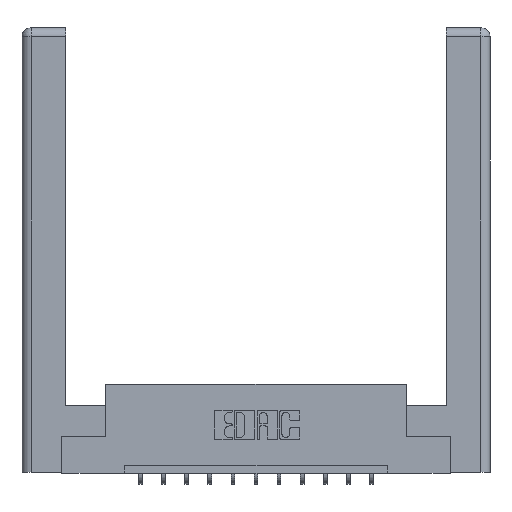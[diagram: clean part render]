
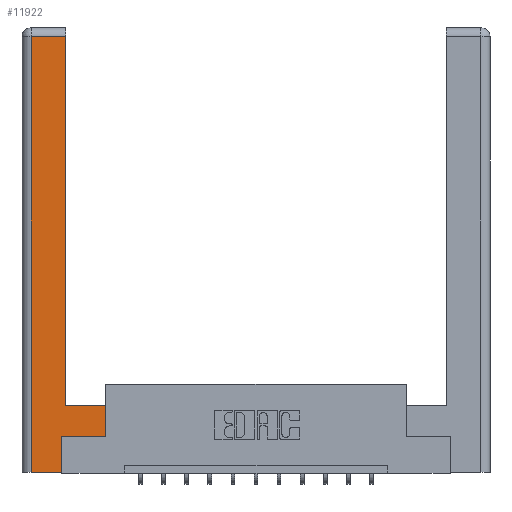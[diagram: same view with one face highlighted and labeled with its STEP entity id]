
A CAD part, top view. The second image highlights one B-rep face of the part: STEP entity #11922.
In plain terms, the highlighted planar face has unit normal (0, 0, 1).
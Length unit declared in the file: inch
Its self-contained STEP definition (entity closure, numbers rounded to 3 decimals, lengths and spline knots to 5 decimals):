
#155 = ORIENTED_EDGE ( 'NONE', *, *, #1983, .T. ) ;
#216 = EDGE_CURVE ( 'NONE', #11898, #9061, #6064, .T. ) ;
#278 = EDGE_CURVE ( 'NONE', #13095, #4959, #3522, .T. ) ;
#535 = PLANE ( 'NONE',  #10379 ) ;
#546 = ORIENTED_EDGE ( 'NONE', *, *, #6426, .T. ) ;
#681 = DIRECTION ( 'NONE',  ( -1., 0., 0. ) ) ;
#907 = CARTESIAN_POINT ( 'NONE',  ( 0.265, 0.245, 0. ) ) ;
#1256 = EDGE_CURVE ( 'NONE', #12566, #13095, #13762, .T. ) ;
#1259 = ORIENTED_EDGE ( 'NONE', *, *, #216, .T. ) ;
#1589 = EDGE_CURVE ( 'NONE', #9061, #14347, #6379, .T. ) ;
#1629 = EDGE_CURVE ( 'NONE', #4959, #14863, #1869, .T. ) ;
#1869 = LINE ( 'NONE', #5887, #4027 ) ;
#1983 = EDGE_CURVE ( 'NONE', #14863, #11898, #4887, .T. ) ;
#2115 = ORIENTED_EDGE ( 'NONE', *, *, #12660, .T. ) ;
#2237 = VECTOR ( 'NONE', #6340, 39.37008 ) ;
#2335 = CARTESIAN_POINT ( 'NONE',  ( 0.565, 0.245, 0. ) ) ;
#2528 = DIRECTION ( 'NONE',  ( 1., 0., 0. ) ) ;
#2892 = CARTESIAN_POINT ( 'NONE',  ( 0.295, 3., 0. ) ) ;
#2978 = CARTESIAN_POINT ( 'NONE',  ( 0.565, 0.45, 0. ) ) ;
#3522 = LINE ( 'NONE', #5352, #13438 ) ;
#3550 = CARTESIAN_POINT ( 'NONE',  ( 0.565, 0.45, 0. ) ) ;
#3569 = CARTESIAN_POINT ( 'NONE',  ( 0.565, 0.245, 0. ) ) ;
#4007 = CARTESIAN_POINT ( 'NONE',  ( 0., 0., 0. ) ) ;
#4027 = VECTOR ( 'NONE', #5947, 39.37008 ) ;
#4887 = LINE ( 'NONE', #9554, #5427 ) ;
#4959 = VERTEX_POINT ( 'NONE', #14123 ) ;
#5352 = CARTESIAN_POINT ( 'NONE',  ( 0.0615, 2.94, 0. ) ) ;
#5427 = VECTOR ( 'NONE', #2528, 39.37008 ) ;
#5678 = CARTESIAN_POINT ( 'NONE',  ( 0.295, 2.94, 0. ) ) ;
#5887 = CARTESIAN_POINT ( 'NONE',  ( 0.0615, 0., 0. ) ) ;
#5947 = DIRECTION ( 'NONE',  ( 0., -1., 0. ) ) ;
#6064 = LINE ( 'NONE', #907, #11830 ) ;
#6340 = DIRECTION ( 'NONE',  ( 0., 1., 0. ) ) ;
#6375 = ORIENTED_EDGE ( 'NONE', *, *, #1589, .T. ) ;
#6379 = LINE ( 'NONE', #3569, #10162 ) ;
#6426 = EDGE_CURVE ( 'NONE', #14347, #8502, #10406, .T. ) ;
#6488 = DIRECTION ( 'NONE',  ( -1., 0., 0. ) ) ;
#6693 = CARTESIAN_POINT ( 'NONE',  ( 0.0615, 0., 0. ) ) ;
#7174 = LINE ( 'NONE', #12273, #10976 ) ;
#7318 = CARTESIAN_POINT ( 'NONE',  ( 0.295, 0.45, 0. ) ) ;
#7627 = DIRECTION ( 'NONE',  ( -1., 0., 0. ) ) ;
#7738 = ORIENTED_EDGE ( 'NONE', *, *, #278, .T. ) ;
#7874 = CARTESIAN_POINT ( 'NONE',  ( 0.265, 0.245, 0. ) ) ;
#7881 = CARTESIAN_POINT ( 'NONE',  ( 0.265, 0., 0. ) ) ;
#8232 = VECTOR ( 'NONE', #12122, 39.37008 ) ;
#8502 = VERTEX_POINT ( 'NONE', #3550 ) ;
#8596 = DIRECTION ( 'NONE',  ( 0., 0., -1. ) ) ;
#9061 = VERTEX_POINT ( 'NONE', #7874 ) ;
#9554 = CARTESIAN_POINT ( 'NONE',  ( 0.265, 0., 0. ) ) ;
#10162 = VECTOR ( 'NONE', #12833, 39.37008 ) ;
#10379 = AXIS2_PLACEMENT_3D ( 'NONE', #4007, #8596, #7627 ) ;
#10406 = LINE ( 'NONE', #2978, #8232 ) ;
#10722 = ORIENTED_EDGE ( 'NONE', *, *, #1256, .T. ) ;
#10976 = VECTOR ( 'NONE', #681, 39.37008 ) ;
#11185 = FACE_OUTER_BOUND ( 'NONE', #12816, .T. ) ;
#11230 = ORIENTED_EDGE ( 'NONE', *, *, #1629, .T. ) ;
#11830 = VECTOR ( 'NONE', #14614, 39.37008 ) ;
#11898 = VERTEX_POINT ( 'NONE', #7881 ) ;
#11922 = ADVANCED_FACE ( 'NONE', ( #11185 ), #535, .F. ) ;
#12122 = DIRECTION ( 'NONE',  ( 0., 1., 0. ) ) ;
#12273 = CARTESIAN_POINT ( 'NONE',  ( 0.295, 0.45, 0. ) ) ;
#12566 = VERTEX_POINT ( 'NONE', #7318 ) ;
#12660 = EDGE_CURVE ( 'NONE', #8502, #12566, #7174, .T. ) ;
#12816 = EDGE_LOOP ( 'NONE', ( #10722, #7738, #11230, #155, #1259, #6375, #546, #2115 ) ) ;
#12833 = DIRECTION ( 'NONE',  ( 1., 0., 0. ) ) ;
#13095 = VERTEX_POINT ( 'NONE', #5678 ) ;
#13438 = VECTOR ( 'NONE', #6488, 39.37008 ) ;
#13762 = LINE ( 'NONE', #2892, #2237 ) ;
#14123 = CARTESIAN_POINT ( 'NONE',  ( 0.0615, 2.94, 0. ) ) ;
#14347 = VERTEX_POINT ( 'NONE', #2335 ) ;
#14614 = DIRECTION ( 'NONE',  ( 0., 1., 0. ) ) ;
#14863 = VERTEX_POINT ( 'NONE', #6693 ) ;
